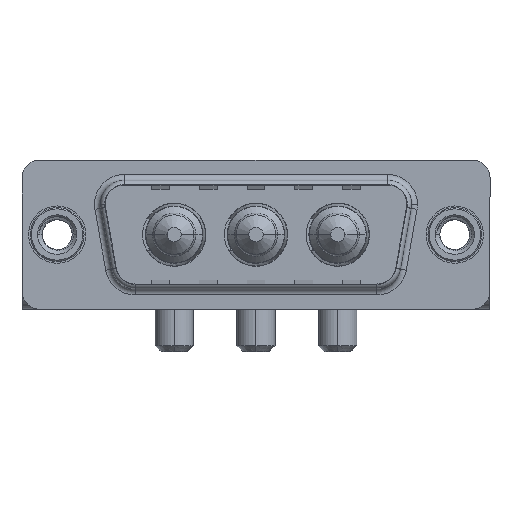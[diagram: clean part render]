
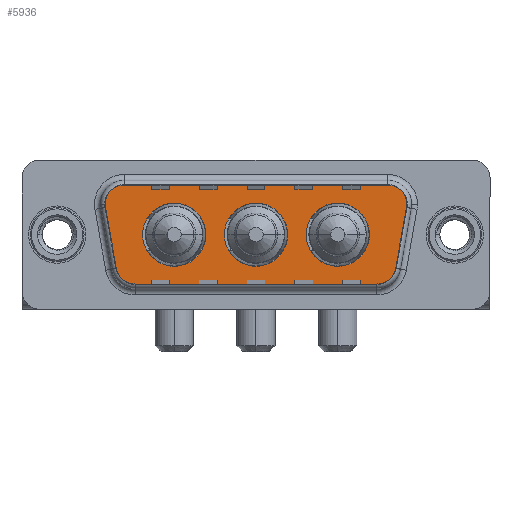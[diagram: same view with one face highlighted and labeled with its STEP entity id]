
A CAD part, top view. The second image highlights one B-rep face of the part: STEP entity #5936.
In plain terms, the highlighted planar face has unit normal (0, 0, 1).
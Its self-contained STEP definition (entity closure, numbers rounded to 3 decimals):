
#132 = AXIS2_PLACEMENT_3D ( 'NONE', #13003, #6067, #381 ) ;
#150 = CARTESIAN_POINT ( 'NONE',  ( 12.45, 0., 0. ) ) ;
#196 = AXIS2_PLACEMENT_3D ( 'NONE', #5960, #9466, #13044 ) ;
#295 = DIRECTION ( 'NONE',  ( 0., 0., 1. ) ) ;
#381 = DIRECTION ( 'NONE',  ( 1., 0., 0. ) ) ;
#383 = DIRECTION ( 'NONE',  ( 1., 0., 0. ) ) ;
#561 = CARTESIAN_POINT ( 'NONE',  ( 7.15, 0., 0. ) ) ;
#678 = CIRCLE ( 'NONE', #2932, 2. ) ;
#1113 = FACE_BOUND ( 'NONE', #14249, .T. ) ;
#1166 = EDGE_CURVE ( 'NONE', #7377, #13286, #13800, .T. ) ;
#2095 = VERTEX_POINT ( 'NONE', #12739 ) ;
#2194 = VERTEX_POINT ( 'NONE', #7985 ) ;
#2270 = CARTESIAN_POINT ( 'NONE',  ( 26.866, -4.9, 0. ) ) ;
#2325 = VECTOR ( 'NONE', #5737, 1000. ) ;
#2364 = DIRECTION ( 'NONE',  ( 0.174, -0.985, 0. ) ) ;
#2388 = DIRECTION ( 'NONE',  ( 0., 0., 1. ) ) ;
#2867 = CARTESIAN_POINT ( 'NONE',  ( 9.8, 0., 0. ) ) ;
#2901 = CARTESIAN_POINT ( 'NONE',  ( 20.85, 0., 0. ) ) ;
#2908 = CARTESIAN_POINT ( 'NONE',  ( 29.859, 2.553, 0. ) ) ;
#2932 = AXIS2_PLACEMENT_3D ( 'NONE', #9027, #14948, #12680 ) ;
#2957 = CIRCLE ( 'NONE', #13126, 2.65 ) ;
#3026 = CARTESIAN_POINT ( 'NONE',  ( 26.15, 0., 0. ) ) ;
#3088 = AXIS2_PLACEMENT_3D ( 'NONE', #7195, #2388, #9455 ) ;
#3155 = CARTESIAN_POINT ( 'NONE',  ( 3.441, 2.553, 0. ) ) ;
#3416 = EDGE_CURVE ( 'NONE', #3860, #12786, #12242, .T. ) ;
#3481 = EDGE_CURVE ( 'NONE', #11324, #9074, #6984, .T. ) ;
#3507 = VERTEX_POINT ( 'NONE', #9470 ) ;
#3584 = EDGE_LOOP ( 'NONE', ( #14626, #11644 ) ) ;
#3623 = EDGE_LOOP ( 'NONE', ( #11722, #7843 ) ) ;
#3860 = VERTEX_POINT ( 'NONE', #3026 ) ;
#3875 = DIRECTION ( 'NONE',  ( 1., 0., 0. ) ) ;
#3899 = ORIENTED_EDGE ( 'NONE', *, *, #14754, .T. ) ;
#4152 = CIRCLE ( 'NONE', #4891, 2.65 ) ;
#4181 = EDGE_CURVE ( 'NONE', #2095, #12900, #11266, .T. ) ;
#4255 = CARTESIAN_POINT ( 'NONE',  ( 29.859, 2.553, 0. ) ) ;
#4420 = VERTEX_POINT ( 'NONE', #11321 ) ;
#4891 = AXIS2_PLACEMENT_3D ( 'NONE', #13779, #12445, #6459 ) ;
#5350 = LINE ( 'NONE', #7836, #15117 ) ;
#5354 = DIRECTION ( 'NONE',  ( 0., 0., 1. ) ) ;
#5365 = CARTESIAN_POINT ( 'NONE',  ( 26.866, -2.9, 0. ) ) ;
#5402 = CIRCLE ( 'NONE', #6910, 2. ) ;
#5737 = DIRECTION ( 'NONE',  ( 1., 0., 0. ) ) ;
#5779 = LINE ( 'NONE', #2908, #8227 ) ;
#5848 = FACE_BOUND ( 'NONE', #3623, .T. ) ;
#5936 = ADVANCED_FACE ( 'NONE', ( #11766, #1113, #5848, #8247 ), #10600, .T. ) ;
#5960 = CARTESIAN_POINT ( 'NONE',  ( 27.889, 2.9, 0. ) ) ;
#6067 = DIRECTION ( 'NONE',  ( 0., 0., 1. ) ) ;
#6140 = CARTESIAN_POINT ( 'NONE',  ( 23.5, 0., 0. ) ) ;
#6156 = EDGE_CURVE ( 'NONE', #9074, #4420, #13050, .T. ) ;
#6459 = DIRECTION ( 'NONE',  ( 1., 0., 0. ) ) ;
#6910 = AXIS2_PLACEMENT_3D ( 'NONE', #12119, #295, #13375 ) ;
#6984 = LINE ( 'NONE', #15168, #2325 ) ;
#7195 = CARTESIAN_POINT ( 'NONE',  ( 27.889, 2.9, 0. ) ) ;
#7219 = VECTOR ( 'NONE', #2364, 1000. ) ;
#7275 = CARTESIAN_POINT ( 'NONE',  ( 27.889, 4.9, 0. ) ) ;
#7377 = VERTEX_POINT ( 'NONE', #11055 ) ;
#7388 = CIRCLE ( 'NONE', #196, 2. ) ;
#7479 = EDGE_CURVE ( 'NONE', #15248, #12132, #4152, .T. ) ;
#7515 = AXIS2_PLACEMENT_3D ( 'NONE', #11276, #5354, #7604 ) ;
#7539 = DIRECTION ( 'NONE',  ( 0., 0., 1. ) ) ;
#7604 = DIRECTION ( 'NONE',  ( 1., 0., 0. ) ) ;
#7836 = CARTESIAN_POINT ( 'NONE',  ( 5.411, 4.9, 0. ) ) ;
#7843 = ORIENTED_EDGE ( 'NONE', *, *, #11709, .F. ) ;
#7852 = DIRECTION ( 'NONE',  ( 0., 0., 1. ) ) ;
#7919 = CARTESIAN_POINT ( 'NONE',  ( 6.434, -4.9, 0. ) ) ;
#7985 = CARTESIAN_POINT ( 'NONE',  ( 14., 0., 0. ) ) ;
#8227 = VECTOR ( 'NONE', #10992, 1000. ) ;
#8247 = FACE_OUTER_BOUND ( 'NONE', #10855, .T. ) ;
#8409 = AXIS2_PLACEMENT_3D ( 'NONE', #2867, #13197, #3875 ) ;
#8516 = VERTEX_POINT ( 'NONE', #4255 ) ;
#8866 = AXIS2_PLACEMENT_3D ( 'NONE', #6140, #7539, #383 ) ;
#8923 = ORIENTED_EDGE ( 'NONE', *, *, #9916, .F. ) ;
#9027 = CARTESIAN_POINT ( 'NONE',  ( 5.411, 2.9, 0. ) ) ;
#9074 = VERTEX_POINT ( 'NONE', #2270 ) ;
#9220 = ORIENTED_EDGE ( 'NONE', *, *, #10445, .T. ) ;
#9277 = DIRECTION ( 'NONE',  ( 1., 0., 0. ) ) ;
#9338 = VERTEX_POINT ( 'NONE', #14383 ) ;
#9372 = CIRCLE ( 'NONE', #8866, 2.65 ) ;
#9380 = ORIENTED_EDGE ( 'NONE', *, *, #4181, .T. ) ;
#9455 = DIRECTION ( 'NONE',  ( -1., 0., 0. ) ) ;
#9466 = DIRECTION ( 'NONE',  ( 0., 0., 1. ) ) ;
#9470 = CARTESIAN_POINT ( 'NONE',  ( 5.411, 4.9, 0. ) ) ;
#9680 = ORIENTED_EDGE ( 'NONE', *, *, #3481, .T. ) ;
#9904 = CARTESIAN_POINT ( 'NONE',  ( 16.65, 0., 0. ) ) ;
#9916 = EDGE_CURVE ( 'NONE', #12786, #3860, #9372, .T. ) ;
#10048 = EDGE_CURVE ( 'NONE', #3507, #7377, #678, .T. ) ;
#10109 = DIRECTION ( 'NONE',  ( 1., 0., 0. ) ) ;
#10445 = EDGE_CURVE ( 'NONE', #13286, #11324, #5402, .T. ) ;
#10451 = CARTESIAN_POINT ( 'NONE',  ( 16.65, 0., 0. ) ) ;
#10504 = EDGE_CURVE ( 'NONE', #12900, #3507, #5350, .T. ) ;
#10600 = PLANE ( 'NONE',  #132 ) ;
#10654 = EDGE_CURVE ( 'NONE', #8516, #2095, #7388, .T. ) ;
#10659 = ORIENTED_EDGE ( 'NONE', *, *, #10048, .T. ) ;
#10855 = EDGE_LOOP ( 'NONE', ( #13866, #3899, #14879, #9380, #14736, #10659, #12612, #9220, #9680 ) ) ;
#10992 = DIRECTION ( 'NONE',  ( 0.174, 0.985, 0. ) ) ;
#11039 = EDGE_CURVE ( 'NONE', #9338, #2194, #2957, .T. ) ;
#11055 = CARTESIAN_POINT ( 'NONE',  ( 3.441, 2.553, 0. ) ) ;
#11152 = CIRCLE ( 'NONE', #8409, 2.65 ) ;
#11156 = DIRECTION ( 'NONE',  ( 0., 0., 1. ) ) ;
#11266 = CIRCLE ( 'NONE', #3088, 2. ) ;
#11276 = CARTESIAN_POINT ( 'NONE',  ( 23.5, 0., 0. ) ) ;
#11321 = CARTESIAN_POINT ( 'NONE',  ( 28.836, -3.247, 0. ) ) ;
#11324 = VERTEX_POINT ( 'NONE', #7919 ) ;
#11644 = ORIENTED_EDGE ( 'NONE', *, *, #13518, .F. ) ;
#11709 = EDGE_CURVE ( 'NONE', #12132, #15248, #11152, .T. ) ;
#11722 = ORIENTED_EDGE ( 'NONE', *, *, #7479, .F. ) ;
#11766 = FACE_BOUND ( 'NONE', #3584, .T. ) ;
#12042 = AXIS2_PLACEMENT_3D ( 'NONE', #5365, #7852, #10109 ) ;
#12119 = CARTESIAN_POINT ( 'NONE',  ( 6.434, -2.9, 0. ) ) ;
#12132 = VERTEX_POINT ( 'NONE', #561 ) ;
#12242 = CIRCLE ( 'NONE', #7515, 2.65 ) ;
#12445 = DIRECTION ( 'NONE',  ( 0., 0., 1. ) ) ;
#12612 = ORIENTED_EDGE ( 'NONE', *, *, #1166, .T. ) ;
#12680 = DIRECTION ( 'NONE',  ( 1., 0., 0. ) ) ;
#12739 = CARTESIAN_POINT ( 'NONE',  ( 29.889, 2.9, 0. ) ) ;
#12786 = VERTEX_POINT ( 'NONE', #2901 ) ;
#12795 = CARTESIAN_POINT ( 'NONE',  ( 4.464, -3.247, 0. ) ) ;
#12900 = VERTEX_POINT ( 'NONE', #7275 ) ;
#13003 = CARTESIAN_POINT ( 'NONE',  ( 26.866, -2.9, 0. ) ) ;
#13044 = DIRECTION ( 'NONE',  ( -1., 0., 0. ) ) ;
#13050 = CIRCLE ( 'NONE', #12042, 2. ) ;
#13126 = AXIS2_PLACEMENT_3D ( 'NONE', #10451, #15209, #9277 ) ;
#13197 = DIRECTION ( 'NONE',  ( 0., 0., 1. ) ) ;
#13286 = VERTEX_POINT ( 'NONE', #12795 ) ;
#13335 = DIRECTION ( 'NONE',  ( 1., 0., 0. ) ) ;
#13375 = DIRECTION ( 'NONE',  ( -1., 0., 0. ) ) ;
#13441 = ORIENTED_EDGE ( 'NONE', *, *, #3416, .F. ) ;
#13518 = EDGE_CURVE ( 'NONE', #2194, #9338, #13932, .T. ) ;
#13605 = DIRECTION ( 'NONE',  ( -1., 0., 0. ) ) ;
#13779 = CARTESIAN_POINT ( 'NONE',  ( 9.8, 0., 0. ) ) ;
#13800 = LINE ( 'NONE', #3155, #7219 ) ;
#13866 = ORIENTED_EDGE ( 'NONE', *, *, #6156, .T. ) ;
#13932 = CIRCLE ( 'NONE', #15182, 2.65 ) ;
#14249 = EDGE_LOOP ( 'NONE', ( #13441, #8923 ) ) ;
#14383 = CARTESIAN_POINT ( 'NONE',  ( 19.3, 0., 0. ) ) ;
#14626 = ORIENTED_EDGE ( 'NONE', *, *, #11039, .F. ) ;
#14736 = ORIENTED_EDGE ( 'NONE', *, *, #10504, .T. ) ;
#14754 = EDGE_CURVE ( 'NONE', #4420, #8516, #5779, .T. ) ;
#14879 = ORIENTED_EDGE ( 'NONE', *, *, #10654, .T. ) ;
#14948 = DIRECTION ( 'NONE',  ( 0., 0., 1. ) ) ;
#15117 = VECTOR ( 'NONE', #13605, 1000. ) ;
#15168 = CARTESIAN_POINT ( 'NONE',  ( 6.434, -4.9, 0. ) ) ;
#15182 = AXIS2_PLACEMENT_3D ( 'NONE', #9904, #11156, #13335 ) ;
#15209 = DIRECTION ( 'NONE',  ( 0., 0., 1. ) ) ;
#15248 = VERTEX_POINT ( 'NONE', #150 ) ;
